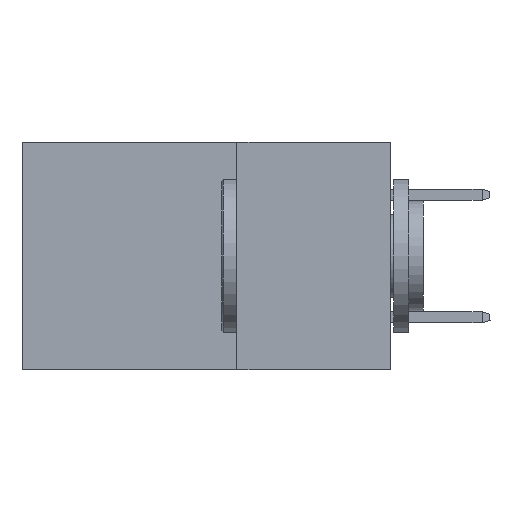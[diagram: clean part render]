
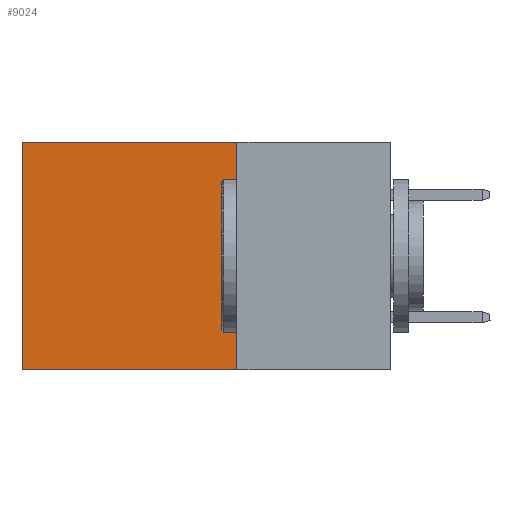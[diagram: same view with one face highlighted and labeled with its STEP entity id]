
A CAD part, left-side view. The second image highlights one B-rep face of the part: STEP entity #9024.
In plain terms, the highlighted planar face has unit normal (-1, 0, 0).
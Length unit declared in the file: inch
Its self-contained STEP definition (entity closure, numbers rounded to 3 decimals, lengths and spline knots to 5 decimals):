
#164 = EDGE_LOOP ( 'NONE', ( #8882, #29147, #2968, #15085 ) ) ;
#2488 = EDGE_CURVE ( 'NONE', #20996, #21427, #5687, .T. ) ;
#2968 = ORIENTED_EDGE ( 'NONE', *, *, #9813, .F. ) ;
#4340 = CARTESIAN_POINT ( 'NONE',  ( 0.2875, 0.25, 0. ) ) ;
#4721 = LINE ( 'NONE', #12684, #13155 ) ;
#5170 = DIRECTION ( 'NONE',  ( 1., 0., 0. ) ) ;
#5687 = LINE ( 'NONE', #4340, #32014 ) ;
#7560 = DIRECTION ( 'NONE',  ( 0., 0., -1. ) ) ;
#7932 = CARTESIAN_POINT ( 'NONE',  ( 0.2875, 0.25, 0. ) ) ;
#8882 = ORIENTED_EDGE ( 'NONE', *, *, #25240, .T. ) ;
#9024 = ADVANCED_FACE ( 'NONE', ( #17913 ), #30421, .F. ) ;
#9104 = CARTESIAN_POINT ( 'NONE',  ( 0.2875, 0.25, 0. ) ) ;
#9537 = CARTESIAN_POINT ( 'NONE',  ( 0.2875, 0.25, -0.37 ) ) ;
#9703 = LINE ( 'NONE', #9537, #10532 ) ;
#9813 = EDGE_CURVE ( 'NONE', #20996, #18440, #11515, .T. ) ;
#9916 = VERTEX_POINT ( 'NONE', #21801 ) ;
#10532 = VECTOR ( 'NONE', #22548, 39.37008 ) ;
#11315 = CARTESIAN_POINT ( 'NONE',  ( 0.2875, 0.25, -0.37 ) ) ;
#11515 = LINE ( 'NONE', #31291, #33009 ) ;
#12684 = CARTESIAN_POINT ( 'NONE',  ( 0.2875, 0.6, 0. ) ) ;
#13155 = VECTOR ( 'NONE', #7560, 39.37008 ) ;
#14490 = DIRECTION ( 'NONE',  ( 0., 0., -1. ) ) ;
#14594 = AXIS2_PLACEMENT_3D ( 'NONE', #9104, #5170, #14490 ) ;
#15085 = ORIENTED_EDGE ( 'NONE', *, *, #2488, .T. ) ;
#15355 = CARTESIAN_POINT ( 'NONE',  ( 0.2875, 0.6, 0. ) ) ;
#15577 = EDGE_CURVE ( 'NONE', #18440, #9916, #9703, .T. ) ;
#17913 = FACE_OUTER_BOUND ( 'NONE', #164, .T. ) ;
#18440 = VERTEX_POINT ( 'NONE', #11315 ) ;
#20996 = VERTEX_POINT ( 'NONE', #7932 ) ;
#21427 = VERTEX_POINT ( 'NONE', #15355 ) ;
#21801 = CARTESIAN_POINT ( 'NONE',  ( 0.2875, 0.6, -0.37 ) ) ;
#22548 = DIRECTION ( 'NONE',  ( 0., 1., 0. ) ) ;
#23710 = DIRECTION ( 'NONE',  ( 0., 0., -1. ) ) ;
#25240 = EDGE_CURVE ( 'NONE', #21427, #9916, #4721, .T. ) ;
#29147 = ORIENTED_EDGE ( 'NONE', *, *, #15577, .F. ) ;
#30421 = PLANE ( 'NONE',  #14594 ) ;
#31291 = CARTESIAN_POINT ( 'NONE',  ( 0.2875, 0.25, 0. ) ) ;
#32014 = VECTOR ( 'NONE', #32016, 39.37008 ) ;
#32016 = DIRECTION ( 'NONE',  ( 0., 1., 0. ) ) ;
#33009 = VECTOR ( 'NONE', #23710, 39.37008 ) ;
